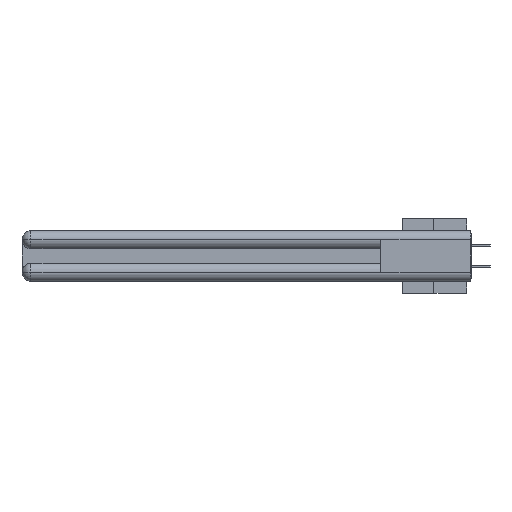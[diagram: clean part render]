
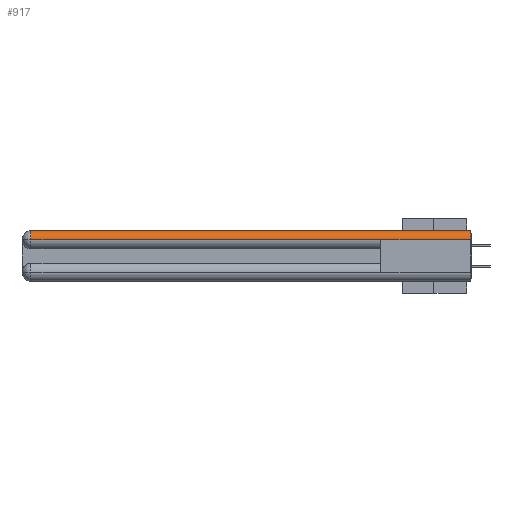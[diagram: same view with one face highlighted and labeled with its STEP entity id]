
A CAD part, left-side view. The second image highlights one B-rep face of the part: STEP entity #917.
In plain terms, the highlighted cylindrical face has radius 1.562 mm (diameter 3.124 mm), a partial arc.
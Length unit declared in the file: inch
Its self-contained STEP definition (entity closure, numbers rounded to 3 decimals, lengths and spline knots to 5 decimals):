
#917 = ADVANCED_FACE ( 'NONE', ( #15378 ), #18609, .T. ) ;
#1527 = EDGE_CURVE ( 'NONE', #33372, #35173, #15785, .T. ) ;
#2529 = AXIS2_PLACEMENT_3D ( 'NONE', #20307, #11086, #5251 ) ;
#2919 = CARTESIAN_POINT ( 'NONE',  ( 0., 2.94, -0.0615 ) ) ;
#3108 = ORIENTED_EDGE ( 'NONE', *, *, #1527, .T. ) ;
#3403 = VERTEX_POINT ( 'NONE', #27514 ) ;
#3828 = VECTOR ( 'NONE', #19603, 39.37008 ) ;
#5251 = DIRECTION ( 'NONE',  ( 1., 0., 0. ) ) ;
#5606 = ORIENTED_EDGE ( 'NONE', *, *, #23930, .F. ) ;
#6129 = LINE ( 'NONE', #34656, #3828 ) ;
#6864 = CARTESIAN_POINT ( 'NONE',  ( 0., 0., -0.0615 ) ) ;
#7595 = DIRECTION ( 'NONE',  ( 0., 1., 0. ) ) ;
#7859 = CARTESIAN_POINT ( 'NONE',  ( 0.0615, 0., -0.0615 ) ) ;
#7983 = VERTEX_POINT ( 'NONE', #6864 ) ;
#8239 = CARTESIAN_POINT ( 'NONE',  ( 0.0615, 2.94, 0. ) ) ;
#9171 = DIRECTION ( 'NONE',  ( 0., -1., 0. ) ) ;
#9361 = VERTEX_POINT ( 'NONE', #8239 ) ;
#10152 = CARTESIAN_POINT ( 'NONE',  ( 0.0615, 2.94, -0.0615 ) ) ;
#11086 = DIRECTION ( 'NONE',  ( 0., -1., 0. ) ) ;
#11489 = VECTOR ( 'NONE', #9171, 39.37008 ) ;
#14726 = DIRECTION ( 'NONE',  ( 0., -1., 0. ) ) ;
#15378 = FACE_OUTER_BOUND ( 'NONE', #17355, .T. ) ;
#15785 = LINE ( 'NONE', #23697, #37103 ) ;
#16569 = LINE ( 'NONE', #23710, #11489 ) ;
#17240 = ORIENTED_EDGE ( 'NONE', *, *, #31069, .F. ) ;
#17355 = EDGE_LOOP ( 'NONE', ( #35747, #17529, #3108, #17240, #5606 ) ) ;
#17356 = EDGE_CURVE ( 'NONE', #9361, #33372, #33892, .T. ) ;
#17529 = ORIENTED_EDGE ( 'NONE', *, *, #17356, .T. ) ;
#18609 = CYLINDRICAL_SURFACE ( 'NONE', #19420, 0.0615 ) ;
#18756 = AXIS2_PLACEMENT_3D ( 'NONE', #10152, #22180, #30901 ) ;
#19094 = EDGE_CURVE ( 'NONE', #9361, #3403, #16569, .T. ) ;
#19420 = AXIS2_PLACEMENT_3D ( 'NONE', #7859, #7595, #37562 ) ;
#19603 = DIRECTION ( 'NONE',  ( 0., 1., 0. ) ) ;
#20307 = CARTESIAN_POINT ( 'NONE',  ( 0.0615, 0., -0.0615 ) ) ;
#22126 = CARTESIAN_POINT ( 'NONE',  ( 0., 0.6, -0.0615 ) ) ;
#22180 = DIRECTION ( 'NONE',  ( 0., -1., 0. ) ) ;
#23697 = CARTESIAN_POINT ( 'NONE',  ( 0., 3., -0.0615 ) ) ;
#23710 = CARTESIAN_POINT ( 'NONE',  ( 0.0615, 0., 0. ) ) ;
#23930 = EDGE_CURVE ( 'NONE', #3403, #7983, #33198, .T. ) ;
#27514 = CARTESIAN_POINT ( 'NONE',  ( 0.0615, 0., 0. ) ) ;
#30901 = DIRECTION ( 'NONE',  ( 0., 0., 1. ) ) ;
#31069 = EDGE_CURVE ( 'NONE', #7983, #35173, #6129, .T. ) ;
#33198 = CIRCLE ( 'NONE', #2529, 0.0615 ) ;
#33372 = VERTEX_POINT ( 'NONE', #2919 ) ;
#33892 = CIRCLE ( 'NONE', #18756, 0.0615 ) ;
#34656 = CARTESIAN_POINT ( 'NONE',  ( 0., 3., -0.0615 ) ) ;
#35173 = VERTEX_POINT ( 'NONE', #22126 ) ;
#35747 = ORIENTED_EDGE ( 'NONE', *, *, #19094, .F. ) ;
#37103 = VECTOR ( 'NONE', #14726, 39.37008 ) ;
#37562 = DIRECTION ( 'NONE',  ( 0., 0., 1. ) ) ;
